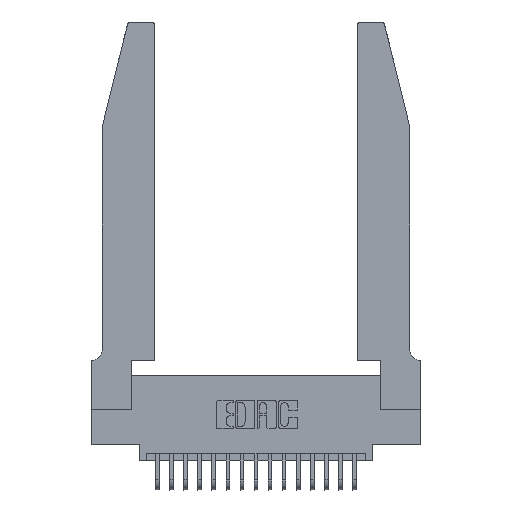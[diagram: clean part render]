
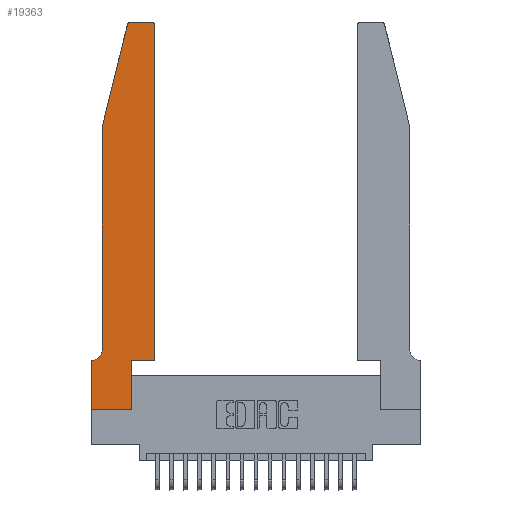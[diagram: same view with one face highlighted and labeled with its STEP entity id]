
A CAD part, top view. The second image highlights one B-rep face of the part: STEP entity #19363.
In plain terms, the highlighted planar face has unit normal (0, 0, 1).
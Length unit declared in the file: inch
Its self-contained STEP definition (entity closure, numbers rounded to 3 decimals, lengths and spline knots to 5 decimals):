
#132 = EDGE_LOOP ( 'NONE', ( #4806, #13928, #12001, #2042, #12504, #141, #11391, #7870, #6083, #12759, #9053, #3650 ) ) ;
#141 = ORIENTED_EDGE ( 'NONE', *, *, #4300, .T. ) ;
#172 = DIRECTION ( 'NONE',  ( 0., 0., 1. ) ) ;
#252 = LINE ( 'NONE', #4375, #17919 ) ;
#392 = VECTOR ( 'NONE', #2322, 39.37008 ) ;
#471 = CARTESIAN_POINT ( 'NONE',  ( 0.0755, 2., 0.37 ) ) ;
#501 = CARTESIAN_POINT ( 'NONE',  ( 0.4505, 0.35, 0.37 ) ) ;
#1191 = VERTEX_POINT ( 'NONE', #7134 ) ;
#1392 = EDGE_CURVE ( 'NONE', #6379, #1191, #4580, .T. ) ;
#1555 = AXIS2_PLACEMENT_3D ( 'NONE', #8267, #9980, #21442 ) ;
#1715 = DIRECTION ( 'NONE',  ( 0., -1., 0. ) ) ;
#1845 = VERTEX_POINT ( 'NONE', #7234 ) ;
#2042 = ORIENTED_EDGE ( 'NONE', *, *, #10367, .T. ) ;
#2106 = CIRCLE ( 'NONE', #13509, 0.03 ) ;
#2124 = LINE ( 'NONE', #12611, #19616 ) ;
#2220 = AXIS2_PLACEMENT_3D ( 'NONE', #11772, #16150, #7991 ) ;
#2284 = DIRECTION ( 'NONE',  ( 0., -1., 0. ) ) ;
#2322 = DIRECTION ( 'NONE',  ( 1., 0., 0. ) ) ;
#2722 = EDGE_CURVE ( 'NONE', #9402, #6379, #12296, .T. ) ;
#3094 = VECTOR ( 'NONE', #11728, 39.37008 ) ;
#3434 = AXIS2_PLACEMENT_3D ( 'NONE', #20190, #10374, #21829 ) ;
#3502 = CARTESIAN_POINT ( 'NONE',  ( 0., 0., 0.37 ) ) ;
#3650 = ORIENTED_EDGE ( 'NONE', *, *, #16564, .T. ) ;
#3961 = EDGE_CURVE ( 'NONE', #11944, #20158, #5021, .T. ) ;
#4113 = EDGE_CURVE ( 'NONE', #12794, #11944, #7241, .T. ) ;
#4300 = EDGE_CURVE ( 'NONE', #17700, #12794, #20708, .T. ) ;
#4375 = CARTESIAN_POINT ( 'NONE',  ( 0.2865, 0.35, 0.37 ) ) ;
#4580 = CIRCLE ( 'NONE', #2220, 0.03 ) ;
#4806 = ORIENTED_EDGE ( 'NONE', *, *, #2722, .T. ) ;
#5021 = LINE ( 'NONE', #18776, #16860 ) ;
#6083 = ORIENTED_EDGE ( 'NONE', *, *, #18085, .T. ) ;
#6379 = VERTEX_POINT ( 'NONE', #14829 ) ;
#6392 = CARTESIAN_POINT ( 'NONE',  ( 0.4505, 0.35, 0.37 ) ) ;
#7134 = CARTESIAN_POINT ( 'NONE',  ( 0.25487, 2.72718, 0.37 ) ) ;
#7234 = CARTESIAN_POINT ( 'NONE',  ( 0.2865, 0.35, 0.37 ) ) ;
#7241 = LINE ( 'NONE', #3502, #15104 ) ;
#7870 = ORIENTED_EDGE ( 'NONE', *, *, #3961, .T. ) ;
#7924 = VERTEX_POINT ( 'NONE', #11223 ) ;
#7991 = DIRECTION ( 'NONE',  ( 1., 0., 0. ) ) ;
#8056 = LINE ( 'NONE', #471, #16366 ) ;
#8088 = DIRECTION ( 'NONE',  ( 0., 1., 0. ) ) ;
#8267 = CARTESIAN_POINT ( 'NONE',  ( 0., 0.35, 0.37 ) ) ;
#8731 = VERTEX_POINT ( 'NONE', #6392 ) ;
#9053 = ORIENTED_EDGE ( 'NONE', *, *, #11072, .T. ) ;
#9402 = VERTEX_POINT ( 'NONE', #18397 ) ;
#9664 = CIRCLE ( 'NONE', #3434, 0.07 ) ;
#9980 = DIRECTION ( 'NONE',  ( 0., 0., 1. ) ) ;
#10057 = CARTESIAN_POINT ( 'NONE',  ( 0.2605, 2.75, 0.37 ) ) ;
#10367 = EDGE_CURVE ( 'NONE', #7924, #14494, #8056, .T. ) ;
#10374 = DIRECTION ( 'NONE',  ( 0., 0., -1. ) ) ;
#10499 = CARTESIAN_POINT ( 'NONE',  ( 0., 0., 0.37 ) ) ;
#10594 = DIRECTION ( 'NONE',  ( 1., 0., 0. ) ) ;
#10720 = CARTESIAN_POINT ( 'NONE',  ( 0.4205, 2.72, 0.37 ) ) ;
#11072 = EDGE_CURVE ( 'NONE', #8731, #15678, #21939, .T. ) ;
#11223 = CARTESIAN_POINT ( 'NONE',  ( 0.0755, 2., 0.37 ) ) ;
#11391 = ORIENTED_EDGE ( 'NONE', *, *, #4113, .T. ) ;
#11545 = CARTESIAN_POINT ( 'NONE',  ( 0.0755, 0.42, 0.37 ) ) ;
#11624 = DIRECTION ( 'NONE',  ( 0., 1., 0. ) ) ;
#11728 = DIRECTION ( 'NONE',  ( -1., 0., 0. ) ) ;
#11772 = CARTESIAN_POINT ( 'NONE',  ( 0.284, 2.72, 0.37 ) ) ;
#11944 = VERTEX_POINT ( 'NONE', #10499 ) ;
#12001 = ORIENTED_EDGE ( 'NONE', *, *, #16178, .T. ) ;
#12118 = CARTESIAN_POINT ( 'NONE',  ( 0.2865, 0., 0.37 ) ) ;
#12296 = LINE ( 'NONE', #10057, #3094 ) ;
#12382 = DIRECTION ( 'NONE',  ( 1., 0., 0. ) ) ;
#12504 = ORIENTED_EDGE ( 'NONE', *, *, #14661, .T. ) ;
#12611 = CARTESIAN_POINT ( 'NONE',  ( 0.0755, 2., 0.37 ) ) ;
#12759 = ORIENTED_EDGE ( 'NONE', *, *, #21692, .T. ) ;
#12794 = VERTEX_POINT ( 'NONE', #20990 ) ;
#13509 = AXIS2_PLACEMENT_3D ( 'NONE', #10720, #172, #12382 ) ;
#13928 = ORIENTED_EDGE ( 'NONE', *, *, #1392, .T. ) ;
#14334 = DIRECTION ( 'NONE',  ( -1., 0., 0. ) ) ;
#14494 = VERTEX_POINT ( 'NONE', #11545 ) ;
#14661 = EDGE_CURVE ( 'NONE', #14494, #17700, #9664, .T. ) ;
#14829 = CARTESIAN_POINT ( 'NONE',  ( 0.284, 2.75, 0.37 ) ) ;
#14847 = CARTESIAN_POINT ( 'NONE',  ( 0.4505, 0.35, 0.37 ) ) ;
#15104 = VECTOR ( 'NONE', #1715, 39.37008 ) ;
#15678 = VERTEX_POINT ( 'NONE', #21002 ) ;
#15922 = CARTESIAN_POINT ( 'NONE',  ( 0.0755, 0.35, 0.37 ) ) ;
#16150 = DIRECTION ( 'NONE',  ( 0., 0., 1. ) ) ;
#16178 = EDGE_CURVE ( 'NONE', #1191, #7924, #2124, .T. ) ;
#16366 = VECTOR ( 'NONE', #2284, 39.37008 ) ;
#16564 = EDGE_CURVE ( 'NONE', #15678, #9402, #2106, .T. ) ;
#16587 = VECTOR ( 'NONE', #11624, 39.37008 ) ;
#16715 = CARTESIAN_POINT ( 'NONE',  ( 0.0055, 0.35, 0.37 ) ) ;
#16860 = VECTOR ( 'NONE', #10594, 39.37008 ) ;
#17432 = DIRECTION ( 'NONE',  ( -0.239, -0.971, 0. ) ) ;
#17700 = VERTEX_POINT ( 'NONE', #16715 ) ;
#17919 = VECTOR ( 'NONE', #8088, 39.37008 ) ;
#18085 = EDGE_CURVE ( 'NONE', #20158, #1845, #252, .T. ) ;
#18169 = PLANE ( 'NONE',  #1555 ) ;
#18397 = CARTESIAN_POINT ( 'NONE',  ( 0.4205, 2.75, 0.37 ) ) ;
#18552 = LINE ( 'NONE', #501, #392 ) ;
#18776 = CARTESIAN_POINT ( 'NONE',  ( 0., 0., 0.37 ) ) ;
#19363 = ADVANCED_FACE ( 'NONE', ( #19912 ), #18169, .T. ) ;
#19616 = VECTOR ( 'NONE', #17432, 39.37008 ) ;
#19912 = FACE_OUTER_BOUND ( 'NONE', #132, .T. ) ;
#20158 = VERTEX_POINT ( 'NONE', #12118 ) ;
#20190 = CARTESIAN_POINT ( 'NONE',  ( 0.0055, 0.42, 0.37 ) ) ;
#20203 = VECTOR ( 'NONE', #14334, 39.37008 ) ;
#20708 = LINE ( 'NONE', #15922, #20203 ) ;
#20990 = CARTESIAN_POINT ( 'NONE',  ( 0., 0.35, 0.37 ) ) ;
#21002 = CARTESIAN_POINT ( 'NONE',  ( 0.4505, 2.72, 0.37 ) ) ;
#21442 = DIRECTION ( 'NONE',  ( 1., 0., 0. ) ) ;
#21692 = EDGE_CURVE ( 'NONE', #1845, #8731, #18552, .T. ) ;
#21829 = DIRECTION ( 'NONE',  ( -1., 0., 0. ) ) ;
#21939 = LINE ( 'NONE', #14847, #16587 ) ;
